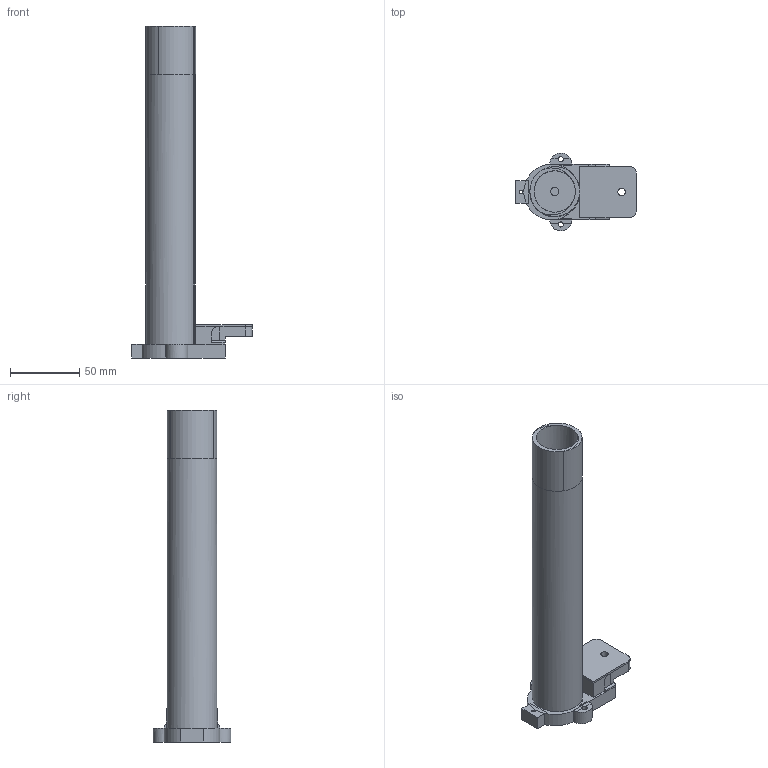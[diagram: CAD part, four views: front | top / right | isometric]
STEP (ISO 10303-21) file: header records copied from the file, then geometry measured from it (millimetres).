
FILE_DESCRIPTION(('FreeCAD Model'),'2;1');
FILE_NAME('ap9 buffer tube pla no support.step','2018-08-08T20:29:04',('Author'),(''), 'Open CASCADE STEP processor 6.8','FreeCAD','Unknown');
FILE_SCHEMA(('AUTOMOTIVE_DESIGN_CC2 { 1 2 10303 214 -1 1 5 4 }'));
Length unit declared in the file: millimetre
Products named in the file (1): Chamfer
Bounding box: 86.94 x 56.2 x 240 mm (x, y, z)
Volume: 164948.2 mm3; surface area: 54772.3 mm2
Topology: 1 solids, 1 shells, 109 faces, 265 edges, 163 vertices
Faces by surface type: plane 75, cylinder 33, cone 1
Full cylindrical faces by diameter (mm): 2.4 x1, 3.7 x2, 5.5 x3, 17.33 x1, 25 x1, 30 x2
Entity records: 6850 total; most frequent: CARTESIAN_POINT 1652, DIRECTION 968, ORIENTED_EDGE 530, PCURVE 530, DEFINITIONAL_REPRESENTATION 530, LINE 488, VECTOR 488, EDGE_CURVE 265
